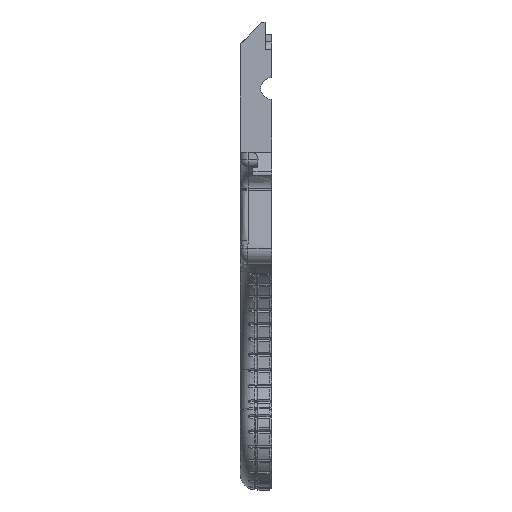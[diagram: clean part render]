
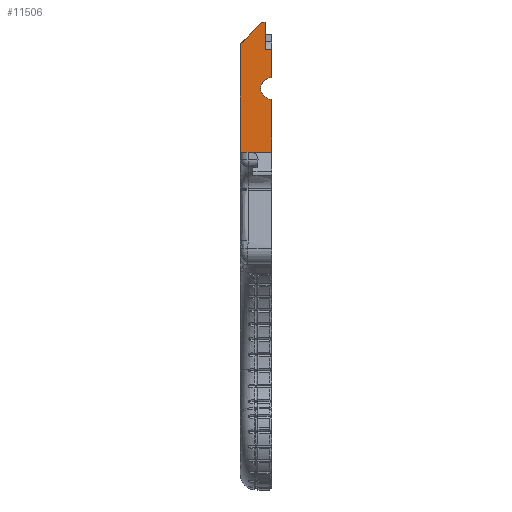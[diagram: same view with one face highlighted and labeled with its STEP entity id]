
A CAD part, top view. The second image highlights one B-rep face of the part: STEP entity #11506.
In plain terms, the highlighted planar face has unit normal (0, 0, 1).
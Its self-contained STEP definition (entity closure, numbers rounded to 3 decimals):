
#46 = CARTESIAN_POINT ( 'NONE',  ( 10., 0., 30.659 ) ) ;
#98 = ORIENTED_EDGE ( 'NONE', *, *, #3870, .F. ) ;
#368 = VECTOR ( 'NONE', #3055, 1000. ) ;
#394 = CARTESIAN_POINT ( 'NONE',  ( 10., 83.24, 30.659 ) ) ;
#1014 = LINE ( 'NONE', #11386, #8511 ) ;
#1028 = CARTESIAN_POINT ( 'NONE',  ( 10., 0., 30.659 ) ) ;
#1163 = EDGE_CURVE ( 'NONE', #12602, #1710, #11647, .T. ) ;
#1710 = VERTEX_POINT ( 'NONE', #18396 ) ;
#1862 = ORIENTED_EDGE ( 'NONE', *, *, #8727, .F. ) ;
#1903 = EDGE_CURVE ( 'NONE', #15071, #12968, #6503, .T. ) ;
#2254 = PLANE ( 'NONE',  #16444 ) ;
#2878 = DIRECTION ( 'NONE',  ( 1., 0., 0. ) ) ;
#2926 = EDGE_CURVE ( 'NONE', #15641, #10782, #14732, .T. ) ;
#3055 = DIRECTION ( 'NONE',  ( 0.707, 0.707, 0. ) ) ;
#3235 = CARTESIAN_POINT ( 'NONE',  ( 10., 76.24, 30.659 ) ) ;
#3311 = DIRECTION ( 'NONE',  ( 0., 1., 0. ) ) ;
#3346 = CARTESIAN_POINT ( 'NONE',  ( 8., 92.24, 30.659 ) ) ;
#3710 = ORIENTED_EDGE ( 'NONE', *, *, #13252, .F. ) ;
#3870 = EDGE_CURVE ( 'NONE', #15035, #11015, #13572, .T. ) ;
#4193 = VECTOR ( 'NONE', #14746, 1000. ) ;
#4365 = DIRECTION ( 'NONE',  ( 0., 1., 0. ) ) ;
#4567 = ORIENTED_EDGE ( 'NONE', *, *, #17690, .T. ) ;
#4844 = ORIENTED_EDGE ( 'NONE', *, *, #13844, .F. ) ;
#5076 = CARTESIAN_POINT ( 'NONE',  ( 10., 59.24, 30.659 ) ) ;
#5190 = CARTESIAN_POINT ( 'NONE',  ( 10., 92.24, 30.659 ) ) ;
#5291 = CARTESIAN_POINT ( 'NONE',  ( 7.414, 100.102, 30.659 ) ) ;
#5354 = ORIENTED_EDGE ( 'NONE', *, *, #14734, .T. ) ;
#5518 = DIRECTION ( 'NONE',  ( 0., 0., 1. ) ) ;
#5816 = VECTOR ( 'NONE', #13588, 1000. ) ;
#5985 = LINE ( 'NONE', #6065, #13097 ) ;
#6065 = CARTESIAN_POINT ( 'NONE',  ( 8., 0., 30.659 ) ) ;
#6156 = CARTESIAN_POINT ( 'NONE',  ( 10., 0., 30.659 ) ) ;
#6301 = VECTOR ( 'NONE', #10437, 1000. ) ;
#6407 = CIRCLE ( 'NONE', #8810, 3.5 ) ;
#6503 = CIRCLE ( 'NONE', #12398, 1. ) ;
#6701 = DIRECTION ( 'NONE',  ( 0., 0., 1. ) ) ;
#6709 = DIRECTION ( 'NONE',  ( 1., 0., 0. ) ) ;
#6872 = ORIENTED_EDGE ( 'NONE', *, *, #1903, .T. ) ;
#6958 = VERTEX_POINT ( 'NONE', #394 ) ;
#7494 = DIRECTION ( 'NONE',  ( 0., -1., 0. ) ) ;
#7950 = LINE ( 'NONE', #18000, #4193 ) ;
#8227 = EDGE_CURVE ( 'NONE', #15641, #11114, #1014, .T. ) ;
#8412 = EDGE_CURVE ( 'NONE', #12968, #1710, #10062, .T. ) ;
#8511 = VECTOR ( 'NONE', #2878, 1000. ) ;
#8727 = EDGE_CURVE ( 'NONE', #10782, #12602, #13891, .T. ) ;
#8810 = AXIS2_PLACEMENT_3D ( 'NONE', #14024, #5518, #15472 ) ;
#9509 = CARTESIAN_POINT ( 'NONE',  ( 3.145, 59.24, 30.659 ) ) ;
#9737 = DIRECTION ( 'NONE',  ( 0., 1., 0. ) ) ;
#9775 = VECTOR ( 'NONE', #10471, 1000. ) ;
#10062 = LINE ( 'NONE', #17546, #6301 ) ;
#10089 = VECTOR ( 'NONE', #9737, 1000. ) ;
#10437 = DIRECTION ( 'NONE',  ( -0.707, -0.707, 0. ) ) ;
#10471 = DIRECTION ( 'NONE',  ( 1., 0., 0. ) ) ;
#10648 = ORIENTED_EDGE ( 'NONE', *, *, #8412, .T. ) ;
#10782 = VERTEX_POINT ( 'NONE', #17500 ) ;
#10920 = VECTOR ( 'NONE', #3311, 1000. ) ;
#11015 = VERTEX_POINT ( 'NONE', #5190 ) ;
#11114 = VERTEX_POINT ( 'NONE', #15258 ) ;
#11361 = LINE ( 'NONE', #6156, #10920 ) ;
#11386 = CARTESIAN_POINT ( 'NONE',  ( 10., 59.24, 30.659 ) ) ;
#11506 = ADVANCED_FACE ( 'NONE', ( #13362 ), #2254, .T. ) ;
#11520 = ORIENTED_EDGE ( 'NONE', *, *, #17919, .T. ) ;
#11564 = CARTESIAN_POINT ( 'NONE',  ( -47.051, 47.051, 30.659 ) ) ;
#11647 = LINE ( 'NONE', #11564, #368 ) ;
#11683 = ORIENTED_EDGE ( 'NONE', *, *, #8227, .T. ) ;
#11975 = CARTESIAN_POINT ( 'NONE',  ( 8., 101.102, 30.659 ) ) ;
#12398 = AXIS2_PLACEMENT_3D ( 'NONE', #5291, #15243, #6709 ) ;
#12550 = CARTESIAN_POINT ( 'NONE',  ( 0., 0., 30.659 ) ) ;
#12602 = VERTEX_POINT ( 'NONE', #15744 ) ;
#12855 = VERTEX_POINT ( 'NONE', #11975 ) ;
#12968 = VERTEX_POINT ( 'NONE', #17981 ) ;
#12994 = ORIENTED_EDGE ( 'NONE', *, *, #1163, .F. ) ;
#13097 = VECTOR ( 'NONE', #7494, 1000. ) ;
#13252 = EDGE_CURVE ( 'NONE', #12855, #15035, #5985, .T. ) ;
#13266 = CARTESIAN_POINT ( 'NONE',  ( 10., 92.24, 30.659 ) ) ;
#13350 = LINE ( 'NONE', #46, #17151 ) ;
#13362 = FACE_OUTER_BOUND ( 'NONE', #16613, .T. ) ;
#13572 = LINE ( 'NONE', #13266, #9775 ) ;
#13588 = DIRECTION ( 'NONE',  ( -1., 0., 0. ) ) ;
#13844 = EDGE_CURVE ( 'NONE', #6958, #16875, #6407, .T. ) ;
#13891 = LINE ( 'NONE', #12550, #10089 ) ;
#14024 = CARTESIAN_POINT ( 'NONE',  ( 10., 79.74, 30.659 ) ) ;
#14729 = CARTESIAN_POINT ( 'NONE',  ( 7.414, 101.102, 30.659 ) ) ;
#14732 = LINE ( 'NONE', #5076, #5816 ) ;
#14734 = EDGE_CURVE ( 'NONE', #12855, #15071, #7950, .T. ) ;
#14746 = DIRECTION ( 'NONE',  ( -1., 0., 0. ) ) ;
#14825 = ORIENTED_EDGE ( 'NONE', *, *, #2926, .F. ) ;
#15035 = VERTEX_POINT ( 'NONE', #3346 ) ;
#15071 = VERTEX_POINT ( 'NONE', #14729 ) ;
#15243 = DIRECTION ( 'NONE',  ( 0., 0., 1. ) ) ;
#15258 = CARTESIAN_POINT ( 'NONE',  ( 10., 59.24, 30.659 ) ) ;
#15472 = DIRECTION ( 'NONE',  ( 1., 0., 0. ) ) ;
#15641 = VERTEX_POINT ( 'NONE', #9509 ) ;
#15744 = CARTESIAN_POINT ( 'NONE',  ( 0., 94.102, 30.659 ) ) ;
#16444 = AXIS2_PLACEMENT_3D ( 'NONE', #1028, #6701, #16666 ) ;
#16613 = EDGE_LOOP ( 'NONE', ( #12994, #1862, #14825, #11683, #4567, #4844, #11520, #98, #3710, #5354, #6872, #10648 ) ) ;
#16666 = DIRECTION ( 'NONE',  ( 1., 0., 0. ) ) ;
#16875 = VERTEX_POINT ( 'NONE', #3235 ) ;
#17151 = VECTOR ( 'NONE', #4365, 1000. ) ;
#17500 = CARTESIAN_POINT ( 'NONE',  ( 0., 59.24, 30.659 ) ) ;
#17546 = CARTESIAN_POINT ( 'NONE',  ( -47.051, 47.051, 30.659 ) ) ;
#17690 = EDGE_CURVE ( 'NONE', #11114, #16875, #11361, .T. ) ;
#17919 = EDGE_CURVE ( 'NONE', #6958, #11015, #13350, .T. ) ;
#17981 = CARTESIAN_POINT ( 'NONE',  ( 6.707, 100.809, 30.659 ) ) ;
#18000 = CARTESIAN_POINT ( 'NONE',  ( 0., 101.102, 30.659 ) ) ;
#18396 = CARTESIAN_POINT ( 'NONE',  ( 0.557, 94.659, 30.659 ) ) ;
